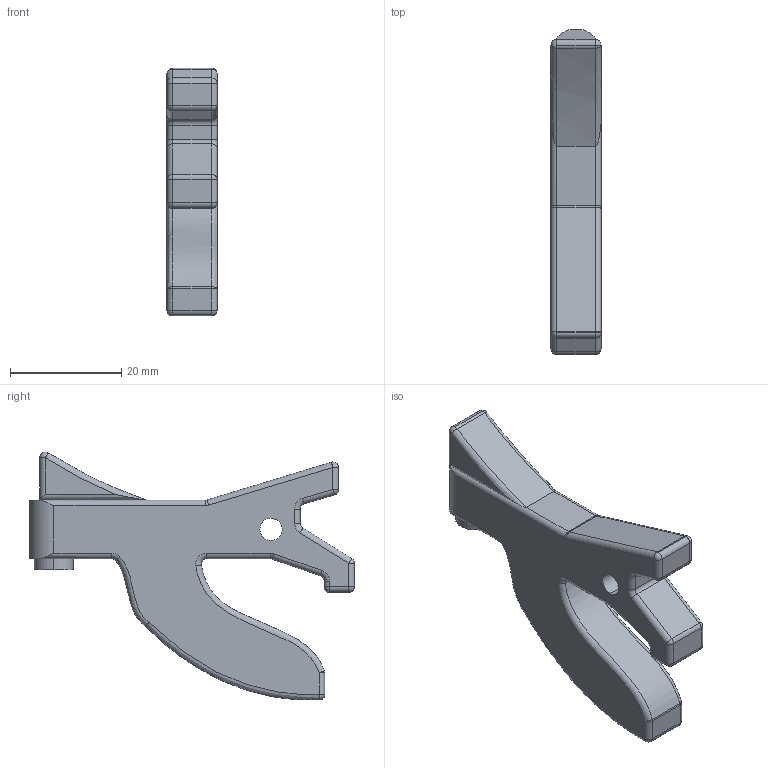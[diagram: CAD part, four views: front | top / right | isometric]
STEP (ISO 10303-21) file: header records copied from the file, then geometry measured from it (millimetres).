
FILE_DESCRIPTION (( 'STEP AP203' ), '1' );
FILE_NAME ('final_hammer_spur.STEP', '2013-07-19T06:22:53', ( '' ), ( '' ), 'SwSTEP 2.0', 'SolidWorks 2012', '' );
FILE_SCHEMA (( 'CONFIG_CONTROL_DESIGN' ));
Length unit declared in the file: millimetre
Products named in the file (1): final_hammer_spur
Bounding box: 9 x 58.36 x 44.5 mm (x, y, z)
Volume: 10809.6 mm3; surface area: 4545.6 mm2
Topology: 1 solids, 1 shells, 121 faces, 279 edges, 144 vertices
Faces by surface type: cylinder 54, plane 23, sphere 18, torus 14, bspline 12
Entity records: 4186 total; most frequent: CARTESIAN_POINT 1503, DIRECTION 581, ORIENTED_EDGE 526, EDGE_CURVE 263, AXIS2_PLACEMENT_3D 234, VERTEX_POINT 144, CIRCLE 124, EDGE_LOOP 123
